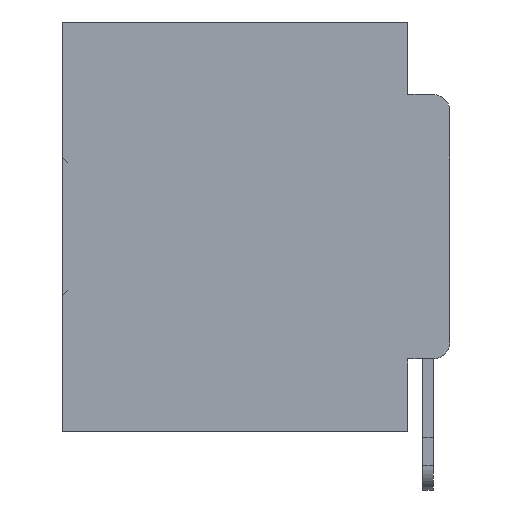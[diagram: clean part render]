
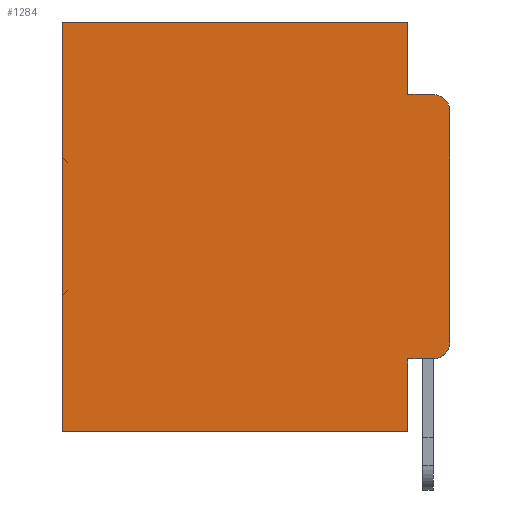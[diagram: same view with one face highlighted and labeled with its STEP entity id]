
A CAD part, left-side view. The second image highlights one B-rep face of the part: STEP entity #1284.
In plain terms, the highlighted planar face has unit normal (-1, 0, 0).
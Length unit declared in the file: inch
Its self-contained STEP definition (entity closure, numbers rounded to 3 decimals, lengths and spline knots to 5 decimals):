
#17 = DIRECTION ( 'NONE',  ( 0., 0., -1. ) ) ;
#161 = DIRECTION ( 'NONE',  ( -1., 0., 0. ) ) ;
#876 = ORIENTED_EDGE ( 'NONE', *, *, #18316, .T. ) ;
#1076 = VECTOR ( 'NONE', #17, 39.37008 ) ;
#1284 = ADVANCED_FACE ( 'NONE', ( #29853 ), #15453, .F. ) ;
#1323 = ORIENTED_EDGE ( 'NONE', *, *, #16607, .F. ) ;
#1757 = CARTESIAN_POINT ( 'NONE',  ( 0.298, 0., 0. ) ) ;
#3199 = EDGE_CURVE ( 'NONE', #9998, #8380, #18448, .T. ) ;
#3244 = DIRECTION ( 'NONE',  ( 0., 0., -1. ) ) ;
#3265 = ORIENTED_EDGE ( 'NONE', *, *, #3199, .T. ) ;
#4377 = CARTESIAN_POINT ( 'NONE',  ( 0.298, 0.473, -0.5 ) ) ;
#4466 = ORIENTED_EDGE ( 'NONE', *, *, #23445, .F. ) ;
#4608 = CARTESIAN_POINT ( 'NONE',  ( 0.298, 0.051, -0.0885 ) ) ;
#5230 = DIRECTION ( 'NONE',  ( 0., 0., -1. ) ) ;
#5603 = VERTEX_POINT ( 'NONE', #20101 ) ;
#6265 = VERTEX_POINT ( 'NONE', #4377 ) ;
#6510 = DIRECTION ( 'NONE',  ( 0., -1., 0. ) ) ;
#7408 = EDGE_CURVE ( 'NONE', #32059, #9038, #7475, .T. ) ;
#7475 = LINE ( 'NONE', #20111, #29040 ) ;
#7649 = CARTESIAN_POINT ( 'NONE',  ( 0.298, 0.051, 0. ) ) ;
#8200 = VECTOR ( 'NONE', #12837, 39.37008 ) ;
#8347 = ORIENTED_EDGE ( 'NONE', *, *, #12479, .F. ) ;
#8380 = VERTEX_POINT ( 'NONE', #34657 ) ;
#8793 = ORIENTED_EDGE ( 'NONE', *, *, #15474, .T. ) ;
#9038 = VERTEX_POINT ( 'NONE', #10535 ) ;
#9321 = VECTOR ( 'NONE', #3244, 39.37008 ) ;
#9998 = VERTEX_POINT ( 'NONE', #14460 ) ;
#10396 = EDGE_CURVE ( 'NONE', #15227, #5603, #19048, .T. ) ;
#10535 = CARTESIAN_POINT ( 'NONE',  ( 0.298, 0.051, -0.0885 ) ) ;
#10781 = CARTESIAN_POINT ( 'NONE',  ( 0.298, 0.051, 0. ) ) ;
#11186 = VECTOR ( 'NONE', #6510, 39.37008 ) ;
#11197 = CARTESIAN_POINT ( 'NONE',  ( 0.298, 0.473, 0. ) ) ;
#11314 = EDGE_CURVE ( 'NONE', #8380, #13848, #19812, .T. ) ;
#11441 = LINE ( 'NONE', #11770, #31185 ) ;
#11770 = CARTESIAN_POINT ( 'NONE',  ( 0.298, 0., -0.5 ) ) ;
#12128 = ORIENTED_EDGE ( 'NONE', *, *, #7408, .F. ) ;
#12479 = EDGE_CURVE ( 'NONE', #9998, #13732, #15172, .T. ) ;
#12595 = VECTOR ( 'NONE', #5230, 39.37008 ) ;
#12837 = DIRECTION ( 'NONE',  ( 0., -1., 0. ) ) ;
#12840 = DIRECTION ( 'NONE',  ( 0., 0., -1. ) ) ;
#13701 = CARTESIAN_POINT ( 'NONE',  ( 0.298, 0.02, -0.1085 ) ) ;
#13732 = VERTEX_POINT ( 'NONE', #22677 ) ;
#13848 = VERTEX_POINT ( 'NONE', #31149 ) ;
#14157 = VERTEX_POINT ( 'NONE', #21696 ) ;
#14460 = CARTESIAN_POINT ( 'NONE',  ( 0.298, 0.051, -0.4115 ) ) ;
#14544 = DIRECTION ( 'NONE',  ( 0., 1., 0. ) ) ;
#14607 = ORIENTED_EDGE ( 'NONE', *, *, #11314, .T. ) ;
#15172 = LINE ( 'NONE', #10781, #12595 ) ;
#15227 = VERTEX_POINT ( 'NONE', #21060 ) ;
#15383 = LINE ( 'NONE', #19940, #20840 ) ;
#15453 = PLANE ( 'NONE',  #21466 ) ;
#15474 = EDGE_CURVE ( 'NONE', #14157, #6265, #18320, .T. ) ;
#16447 = DIRECTION ( 'NONE',  ( 0., 0., -1. ) ) ;
#16607 = EDGE_CURVE ( 'NONE', #9038, #5603, #28916, .T. ) ;
#16745 = CARTESIAN_POINT ( 'NONE',  ( 0.298, 0.02, -0.3915 ) ) ;
#17448 = CARTESIAN_POINT ( 'NONE',  ( 0.298, 0.051, -0.4115 ) ) ;
#18316 = EDGE_CURVE ( 'NONE', #32059, #14157, #15383, .T. ) ;
#18320 = LINE ( 'NONE', #11197, #1076 ) ;
#18448 = LINE ( 'NONE', #17448, #11186 ) ;
#18523 = ORIENTED_EDGE ( 'NONE', *, *, #18883, .F. ) ;
#18883 = EDGE_CURVE ( 'NONE', #15227, #13848, #23777, .T. ) ;
#19048 = CIRCLE ( 'NONE', #20568, 0.02 ) ;
#19428 = DIRECTION ( 'NONE',  ( 0., 0., -1. ) ) ;
#19812 = CIRCLE ( 'NONE', #31079, 0.02 ) ;
#19940 = CARTESIAN_POINT ( 'NONE',  ( 0.298, 0., 0. ) ) ;
#20078 = DIRECTION ( 'NONE',  ( 1., 0., 0. ) ) ;
#20101 = CARTESIAN_POINT ( 'NONE',  ( 0.298, 0.02, -0.0885 ) ) ;
#20111 = CARTESIAN_POINT ( 'NONE',  ( 0.298, 0.051, 0. ) ) ;
#20568 = AXIS2_PLACEMENT_3D ( 'NONE', #13701, #32403, #16447 ) ;
#20840 = VECTOR ( 'NONE', #30561, 39.37008 ) ;
#21060 = CARTESIAN_POINT ( 'NONE',  ( 0.298, 0., -0.1085 ) ) ;
#21466 = AXIS2_PLACEMENT_3D ( 'NONE', #1757, #20078, #12840 ) ;
#21696 = CARTESIAN_POINT ( 'NONE',  ( 0.298, 0.473, 0. ) ) ;
#22677 = CARTESIAN_POINT ( 'NONE',  ( 0.298, 0.051, -0.5 ) ) ;
#22788 = ORIENTED_EDGE ( 'NONE', *, *, #10396, .T. ) ;
#23445 = EDGE_CURVE ( 'NONE', #13732, #6265, #11441, .T. ) ;
#23777 = LINE ( 'NONE', #25099, #9321 ) ;
#25099 = CARTESIAN_POINT ( 'NONE',  ( 0.298, 0., 0. ) ) ;
#27013 = EDGE_LOOP ( 'NONE', ( #18523, #22788, #1323, #12128, #876, #8793, #4466, #8347, #3265, #14607 ) ) ;
#28068 = DIRECTION ( 'NONE',  ( 0., 0., -1. ) ) ;
#28916 = LINE ( 'NONE', #4608, #8200 ) ;
#29040 = VECTOR ( 'NONE', #28068, 39.37008 ) ;
#29853 = FACE_OUTER_BOUND ( 'NONE', #27013, .T. ) ;
#30561 = DIRECTION ( 'NONE',  ( 0., 1., 0. ) ) ;
#31079 = AXIS2_PLACEMENT_3D ( 'NONE', #16745, #161, #19428 ) ;
#31149 = CARTESIAN_POINT ( 'NONE',  ( 0.298, 0., -0.3915 ) ) ;
#31185 = VECTOR ( 'NONE', #14544, 39.37008 ) ;
#32059 = VERTEX_POINT ( 'NONE', #7649 ) ;
#32403 = DIRECTION ( 'NONE',  ( -1., 0., 0. ) ) ;
#34657 = CARTESIAN_POINT ( 'NONE',  ( 0.298, 0.02, -0.4115 ) ) ;
